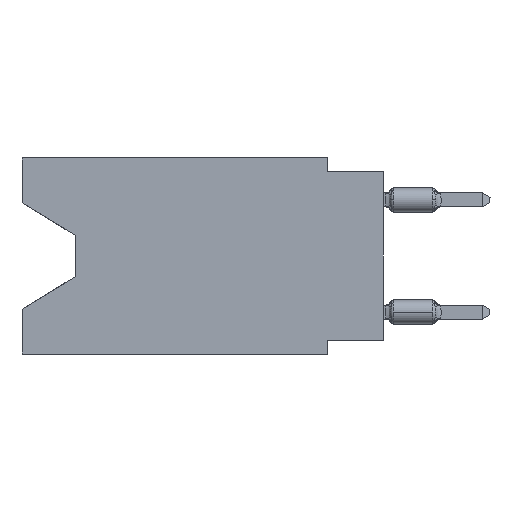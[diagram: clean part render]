
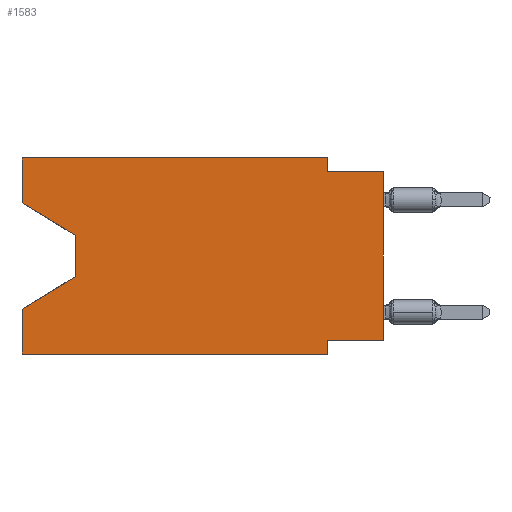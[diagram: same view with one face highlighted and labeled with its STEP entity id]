
A CAD part, left-side view. The second image highlights one B-rep face of the part: STEP entity #1583.
In plain terms, the highlighted planar face has unit normal (-1, 0, 0).
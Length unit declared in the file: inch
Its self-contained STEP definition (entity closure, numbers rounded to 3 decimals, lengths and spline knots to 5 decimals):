
#29 = LINE ( 'NONE', #24904, #1126 ) ;
#704 = DIRECTION ( 'NONE',  ( 0., 0., -1. ) ) ;
#1126 = VECTOR ( 'NONE', #20590, 39.37008 ) ;
#1259 = VERTEX_POINT ( 'NONE', #23724 ) ;
#1260 = CARTESIAN_POINT ( 'NONE',  ( 0., 0.55, -0.138 ) ) ;
#1418 = VECTOR ( 'NONE', #24673, 39.37008 ) ;
#1475 = ORIENTED_EDGE ( 'NONE', *, *, #21198, .T. ) ;
#1583 = ADVANCED_FACE ( 'NONE', ( #18519 ), #25644, .F. ) ;
#1703 = VECTOR ( 'NONE', #20769, 39.37008 ) ;
#2309 = LINE ( 'NONE', #17944, #1703 ) ;
#2388 = CARTESIAN_POINT ( 'NONE',  ( 0., 0., -0.025 ) ) ;
#2896 = CARTESIAN_POINT ( 'NONE',  ( 0., 0., -0.025 ) ) ;
#2949 = LINE ( 'NONE', #21385, #25197 ) ;
#3117 = ORIENTED_EDGE ( 'NONE', *, *, #15672, .F. ) ;
#3167 = LINE ( 'NONE', #2896, #28413 ) ;
#4135 = EDGE_CURVE ( 'NONE', #11732, #18343, #29, .T. ) ;
#4671 = ORIENTED_EDGE ( 'NONE', *, *, #5266, .T. ) ;
#4858 = VECTOR ( 'NONE', #23822, 39.37008 ) ;
#4977 = DIRECTION ( 'NONE',  ( 0., -1., 0. ) ) ;
#5091 = DIRECTION ( 'NONE',  ( 0., -1., 0. ) ) ;
#5266 = EDGE_CURVE ( 'NONE', #11732, #24836, #8450, .T. ) ;
#5818 = CARTESIAN_POINT ( 'NONE',  ( 0., 0.645, -0.08025 ) ) ;
#6011 = EDGE_CURVE ( 'NONE', #20401, #13555, #10719, .T. ) ;
#6023 = EDGE_LOOP ( 'NONE', ( #4671, #1475, #11019, #18600, #11771, #14008, #9064, #20034, #10836, #7231, #3117, #10645 ) ) ;
#6106 = LINE ( 'NONE', #24257, #13032 ) ;
#7231 = ORIENTED_EDGE ( 'NONE', *, *, #13785, .F. ) ;
#8374 = LINE ( 'NONE', #21298, #4858 ) ;
#8415 = LINE ( 'NONE', #8716, #27174 ) ;
#8450 = LINE ( 'NONE', #28951, #11910 ) ;
#8716 = CARTESIAN_POINT ( 'NONE',  ( 0., 0., -0.325 ) ) ;
#9064 = ORIENTED_EDGE ( 'NONE', *, *, #9642, .F. ) ;
#9642 = EDGE_CURVE ( 'NONE', #14485, #20401, #8415, .T. ) ;
#10227 = DIRECTION ( 'NONE',  ( 0., 0., -1. ) ) ;
#10645 = ORIENTED_EDGE ( 'NONE', *, *, #4135, .F. ) ;
#10719 = LINE ( 'NONE', #27050, #1418 ) ;
#10805 = CARTESIAN_POINT ( 'NONE',  ( 0., 0.1, 0. ) ) ;
#10836 = ORIENTED_EDGE ( 'NONE', *, *, #18793, .F. ) ;
#11019 = ORIENTED_EDGE ( 'NONE', *, *, #11191, .T. ) ;
#11191 = EDGE_CURVE ( 'NONE', #24432, #27943, #16916, .T. ) ;
#11313 = VERTEX_POINT ( 'NONE', #10805 ) ;
#11685 = DIRECTION ( 'NONE',  ( 0., 0., -1. ) ) ;
#11732 = VERTEX_POINT ( 'NONE', #5818 ) ;
#11771 = ORIENTED_EDGE ( 'NONE', *, *, #14435, .T. ) ;
#11804 = LINE ( 'NONE', #14155, #18094 ) ;
#11910 = VECTOR ( 'NONE', #22240, 39.37008 ) ;
#12984 = VECTOR ( 'NONE', #25539, 39.37008 ) ;
#13005 = DIRECTION ( 'NONE',  ( 0., 1., 0. ) ) ;
#13032 = VECTOR ( 'NONE', #21730, 39.37008 ) ;
#13291 = VECTOR ( 'NONE', #10227, 39.37008 ) ;
#13555 = VERTEX_POINT ( 'NONE', #15592 ) ;
#13785 = EDGE_CURVE ( 'NONE', #11313, #1259, #2949, .T. ) ;
#14008 = ORIENTED_EDGE ( 'NONE', *, *, #6011, .F. ) ;
#14155 = CARTESIAN_POINT ( 'NONE',  ( 0., 0.645, -0.35 ) ) ;
#14435 = EDGE_CURVE ( 'NONE', #25493, #13555, #11804, .T. ) ;
#14485 = VERTEX_POINT ( 'NONE', #27559 ) ;
#14531 = CARTESIAN_POINT ( 'NONE',  ( 0., 0.55, -0.212 ) ) ;
#15592 = CARTESIAN_POINT ( 'NONE',  ( 0., 0.1, -0.35 ) ) ;
#15672 = EDGE_CURVE ( 'NONE', #18343, #11313, #8374, .T. ) ;
#15767 = AXIS2_PLACEMENT_3D ( 'NONE', #16734, #16129, #11685 ) ;
#16129 = DIRECTION ( 'NONE',  ( 1., 0., 0. ) ) ;
#16734 = CARTESIAN_POINT ( 'NONE',  ( 0., 0.645, 0. ) ) ;
#16916 = LINE ( 'NONE', #27915, #12984 ) ;
#17904 = EDGE_CURVE ( 'NONE', #25493, #27943, #6106, .T. ) ;
#17944 = CARTESIAN_POINT ( 'NONE',  ( 0., 0., 0. ) ) ;
#18094 = VECTOR ( 'NONE', #5091, 39.37008 ) ;
#18343 = VERTEX_POINT ( 'NONE', #23151 ) ;
#18519 = FACE_OUTER_BOUND ( 'NONE', #6023, .T. ) ;
#18600 = ORIENTED_EDGE ( 'NONE', *, *, #17904, .F. ) ;
#18793 = EDGE_CURVE ( 'NONE', #1259, #27056, #3167, .T. ) ;
#20031 = CARTESIAN_POINT ( 'NONE',  ( 0., 0.645, -0.26975 ) ) ;
#20034 = ORIENTED_EDGE ( 'NONE', *, *, #25866, .T. ) ;
#20401 = VERTEX_POINT ( 'NONE', #29365 ) ;
#20590 = DIRECTION ( 'NONE',  ( 0., 0., 1. ) ) ;
#20769 = DIRECTION ( 'NONE',  ( 0., 0., 1. ) ) ;
#21198 = EDGE_CURVE ( 'NONE', #24836, #24432, #21514, .T. ) ;
#21298 = CARTESIAN_POINT ( 'NONE',  ( 0., 0.645, 0. ) ) ;
#21385 = CARTESIAN_POINT ( 'NONE',  ( 0., 0.1, 0. ) ) ;
#21514 = LINE ( 'NONE', #1260, #13291 ) ;
#21730 = DIRECTION ( 'NONE',  ( 0., 0., 1. ) ) ;
#22240 = DIRECTION ( 'NONE',  ( 0., -0.855, -0.519 ) ) ;
#22876 = CARTESIAN_POINT ( 'NONE',  ( 0., 0.645, -0.35 ) ) ;
#23151 = CARTESIAN_POINT ( 'NONE',  ( 0., 0.645, 0. ) ) ;
#23435 = CARTESIAN_POINT ( 'NONE',  ( 0., 0.55, -0.138 ) ) ;
#23724 = CARTESIAN_POINT ( 'NONE',  ( 0., 0.1, -0.025 ) ) ;
#23822 = DIRECTION ( 'NONE',  ( 0., -1., 0. ) ) ;
#24257 = CARTESIAN_POINT ( 'NONE',  ( 0., 0.645, 0. ) ) ;
#24432 = VERTEX_POINT ( 'NONE', #14531 ) ;
#24673 = DIRECTION ( 'NONE',  ( 0., 0., -1. ) ) ;
#24836 = VERTEX_POINT ( 'NONE', #23435 ) ;
#24904 = CARTESIAN_POINT ( 'NONE',  ( 0., 0.645, 0. ) ) ;
#25197 = VECTOR ( 'NONE', #704, 39.37008 ) ;
#25493 = VERTEX_POINT ( 'NONE', #22876 ) ;
#25539 = DIRECTION ( 'NONE',  ( 0., 0.855, -0.519 ) ) ;
#25644 = PLANE ( 'NONE',  #15767 ) ;
#25866 = EDGE_CURVE ( 'NONE', #14485, #27056, #2309, .T. ) ;
#27050 = CARTESIAN_POINT ( 'NONE',  ( 0., 0.1, -0.35 ) ) ;
#27056 = VERTEX_POINT ( 'NONE', #2388 ) ;
#27174 = VECTOR ( 'NONE', #13005, 39.37008 ) ;
#27559 = CARTESIAN_POINT ( 'NONE',  ( 0., 0., -0.325 ) ) ;
#27915 = CARTESIAN_POINT ( 'NONE',  ( 0., 0.55, -0.212 ) ) ;
#27943 = VERTEX_POINT ( 'NONE', #20031 ) ;
#28413 = VECTOR ( 'NONE', #4977, 39.37008 ) ;
#28951 = CARTESIAN_POINT ( 'NONE',  ( 0., 0.645, -0.08025 ) ) ;
#29365 = CARTESIAN_POINT ( 'NONE',  ( 0., 0.1, -0.325 ) ) ;
